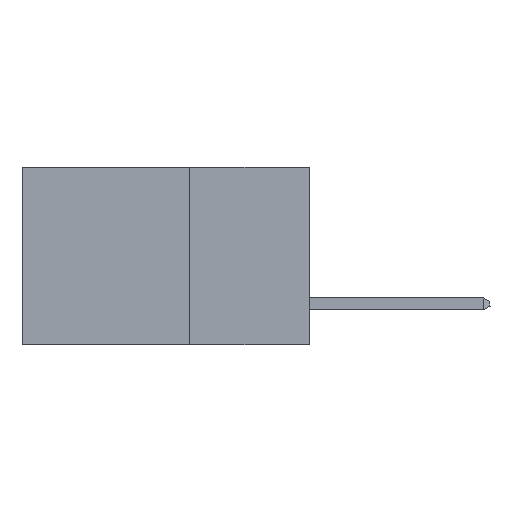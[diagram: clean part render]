
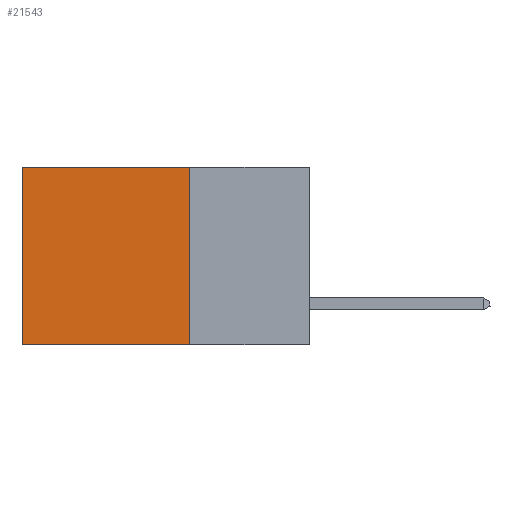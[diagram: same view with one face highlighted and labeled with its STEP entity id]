
A CAD part, left-side view. The second image highlights one B-rep face of the part: STEP entity #21543.
In plain terms, the highlighted planar face has unit normal (-1, 0, 0).
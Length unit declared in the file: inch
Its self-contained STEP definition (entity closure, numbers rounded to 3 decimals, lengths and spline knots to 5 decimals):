
#4705 = DIRECTION ( 'NONE',  ( 0., 1., 0. ) ) ;
#5403 = VERTEX_POINT ( 'NONE', #8046 ) ;
#7342 = CARTESIAN_POINT ( 'NONE',  ( 0.2875, 0.6, 0. ) ) ;
#7350 = VECTOR ( 'NONE', #4705, 39.37008 ) ;
#7696 = LINE ( 'NONE', #18247, #13219 ) ;
#8046 = CARTESIAN_POINT ( 'NONE',  ( 0.2875, 0.6, -0.37 ) ) ;
#8395 = EDGE_CURVE ( 'NONE', #17200, #18488, #10289, .T. ) ;
#9804 = ORIENTED_EDGE ( 'NONE', *, *, #19171, .F. ) ;
#10262 = CARTESIAN_POINT ( 'NONE',  ( 0.2875, 0.25, 0. ) ) ;
#10289 = LINE ( 'NONE', #27696, #21639 ) ;
#11537 = VECTOR ( 'NONE', #20317, 39.37008 ) ;
#12387 = PLANE ( 'NONE',  #27297 ) ;
#13219 = VECTOR ( 'NONE', #13727, 39.37008 ) ;
#13458 = CARTESIAN_POINT ( 'NONE',  ( 0.2875, 0.25, -0.37 ) ) ;
#13474 = EDGE_CURVE ( 'NONE', #17596, #5403, #20529, .T. ) ;
#13727 = DIRECTION ( 'NONE',  ( 0., 1., 0. ) ) ;
#13767 = CARTESIAN_POINT ( 'NONE',  ( 0.2875, 0.25, 0. ) ) ;
#15110 = CARTESIAN_POINT ( 'NONE',  ( 0.2875, 0.6, 0. ) ) ;
#16454 = ORIENTED_EDGE ( 'NONE', *, *, #25063, .T. ) ;
#17200 = VERTEX_POINT ( 'NONE', #13767 ) ;
#17596 = VERTEX_POINT ( 'NONE', #15110 ) ;
#18029 = LINE ( 'NONE', #13458, #7350 ) ;
#18247 = CARTESIAN_POINT ( 'NONE',  ( 0.2875, 0.25, 0. ) ) ;
#18488 = VERTEX_POINT ( 'NONE', #23961 ) ;
#19171 = EDGE_CURVE ( 'NONE', #18488, #5403, #18029, .T. ) ;
#20317 = DIRECTION ( 'NONE',  ( 0., 0., -1. ) ) ;
#20529 = LINE ( 'NONE', #7342, #11537 ) ;
#20987 = FACE_OUTER_BOUND ( 'NONE', #28421, .T. ) ;
#21335 = DIRECTION ( 'NONE',  ( 0., 0., -1. ) ) ;
#21543 = ADVANCED_FACE ( 'NONE', ( #20987 ), #12387, .F. ) ;
#21639 = VECTOR ( 'NONE', #23369, 39.37008 ) ;
#22080 = ORIENTED_EDGE ( 'NONE', *, *, #8395, .F. ) ;
#23369 = DIRECTION ( 'NONE',  ( 0., 0., -1. ) ) ;
#23961 = CARTESIAN_POINT ( 'NONE',  ( 0.2875, 0.25, -0.37 ) ) ;
#25063 = EDGE_CURVE ( 'NONE', #17200, #17596, #7696, .T. ) ;
#25930 = DIRECTION ( 'NONE',  ( 1., 0., 0. ) ) ;
#26731 = ORIENTED_EDGE ( 'NONE', *, *, #13474, .T. ) ;
#27297 = AXIS2_PLACEMENT_3D ( 'NONE', #10262, #25930, #21335 ) ;
#27696 = CARTESIAN_POINT ( 'NONE',  ( 0.2875, 0.25, 0. ) ) ;
#28421 = EDGE_LOOP ( 'NONE', ( #26731, #9804, #22080, #16454 ) ) ;
